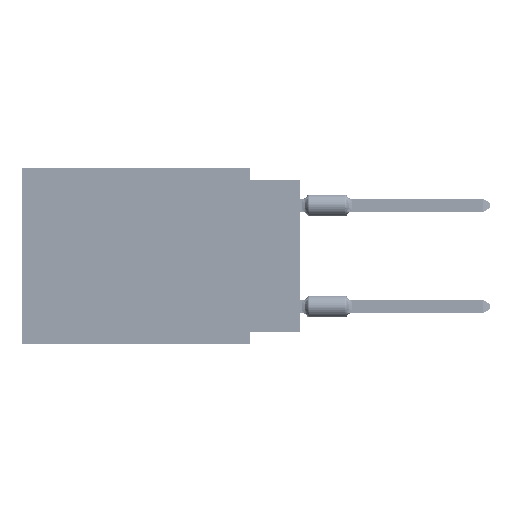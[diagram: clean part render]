
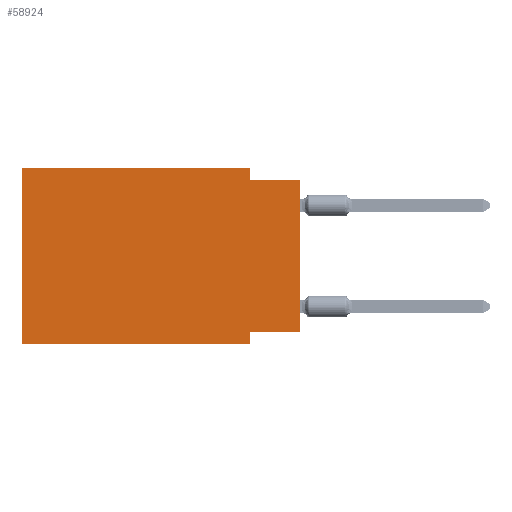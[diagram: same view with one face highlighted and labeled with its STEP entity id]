
A CAD part, left-side view. The second image highlights one B-rep face of the part: STEP entity #58924.
In plain terms, the highlighted planar face has unit normal (-1, 0, 0).
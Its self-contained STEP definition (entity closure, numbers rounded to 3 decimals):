
#3512 = LINE ( 'NONE', #9222, #46817 ) ;
#5720 = EDGE_CURVE ( 'NONE', #57578, #35784, #3512, .T. ) ;
#6951 = CARTESIAN_POINT ( 'NONE',  ( 0., 2.54, -8.255 ) ) ;
#9222 = CARTESIAN_POINT ( 'NONE',  ( 0., 2.54, -8.89 ) ) ;
#10628 = EDGE_LOOP ( 'NONE', ( #24085, #33129, #15882, #14444, #11402, #36207, #34136, #55691 ) ) ;
#11306 = VECTOR ( 'NONE', #19328, 1000. ) ;
#11402 = ORIENTED_EDGE ( 'NONE', *, *, #54731, .F. ) ;
#11644 = VERTEX_POINT ( 'NONE', #34146 ) ;
#11761 = CARTESIAN_POINT ( 'NONE',  ( 0., 13.97, -8.89 ) ) ;
#13430 = VERTEX_POINT ( 'NONE', #50425 ) ;
#13504 = DIRECTION ( 'NONE',  ( 0., -1., 0. ) ) ;
#13558 = VERTEX_POINT ( 'NONE', #47542 ) ;
#14444 = ORIENTED_EDGE ( 'NONE', *, *, #21468, .F. ) ;
#15882 = ORIENTED_EDGE ( 'NONE', *, *, #30518, .F. ) ;
#16103 = EDGE_CURVE ( 'NONE', #55023, #57578, #61866, .T. ) ;
#17272 = CARTESIAN_POINT ( 'NONE',  ( 0., 0., 0. ) ) ;
#17658 = DIRECTION ( 'NONE',  ( 0., -1., 0. ) ) ;
#19060 = EDGE_CURVE ( 'NONE', #11644, #13558, #30659, .T. ) ;
#19328 = DIRECTION ( 'NONE',  ( 0., 1., 0. ) ) ;
#19878 = VECTOR ( 'NONE', #59218, 1000. ) ;
#21468 = EDGE_CURVE ( 'NONE', #13430, #26968, #24415, .T. ) ;
#22025 = LINE ( 'NONE', #64933, #19878 ) ;
#23384 = PLANE ( 'NONE',  #51029 ) ;
#24085 = ORIENTED_EDGE ( 'NONE', *, *, #39243, .T. ) ;
#24415 = LINE ( 'NONE', #46201, #49723 ) ;
#25304 = DIRECTION ( 'NONE',  ( 0., 0., -1. ) ) ;
#26968 = VERTEX_POINT ( 'NONE', #33192 ) ;
#29818 = CARTESIAN_POINT ( 'NONE',  ( 0., 13.97, 0. ) ) ;
#30518 = EDGE_CURVE ( 'NONE', #26968, #11644, #49354, .T. ) ;
#30549 = CARTESIAN_POINT ( 'NONE',  ( 0., 0., -8.255 ) ) ;
#30659 = LINE ( 'NONE', #63192, #38471 ) ;
#33129 = ORIENTED_EDGE ( 'NONE', *, *, #19060, .F. ) ;
#33192 = CARTESIAN_POINT ( 'NONE',  ( 0., 2.54, 0. ) ) ;
#33758 = CARTESIAN_POINT ( 'NONE',  ( 0., 13.97, -8.89 ) ) ;
#34136 = ORIENTED_EDGE ( 'NONE', *, *, #5720, .F. ) ;
#34146 = CARTESIAN_POINT ( 'NONE',  ( 0., 2.54, -0.635 ) ) ;
#35784 = VERTEX_POINT ( 'NONE', #56295 ) ;
#36207 = ORIENTED_EDGE ( 'NONE', *, *, #49438, .T. ) ;
#38471 = VECTOR ( 'NONE', #13504, 1000. ) ;
#38616 = CARTESIAN_POINT ( 'NONE',  ( 0., 2.54, 0. ) ) ;
#39243 = EDGE_CURVE ( 'NONE', #55023, #13558, #44766, .T. ) ;
#42981 = VECTOR ( 'NONE', #17658, 1000. ) ;
#44766 = LINE ( 'NONE', #17272, #67908 ) ;
#45175 = DIRECTION ( 'NONE',  ( 1., 0., 0. ) ) ;
#46201 = CARTESIAN_POINT ( 'NONE',  ( 0., 13.97, 0. ) ) ;
#46817 = VECTOR ( 'NONE', #25304, 1000. ) ;
#47542 = CARTESIAN_POINT ( 'NONE',  ( 0., 0., -0.635 ) ) ;
#49354 = LINE ( 'NONE', #38616, #61385 ) ;
#49438 = EDGE_CURVE ( 'NONE', #62455, #35784, #65937, .T. ) ;
#49723 = VECTOR ( 'NONE', #68030, 1000. ) ;
#50425 = CARTESIAN_POINT ( 'NONE',  ( 0., 13.97, 0. ) ) ;
#51029 = AXIS2_PLACEMENT_3D ( 'NONE', #29818, #45175, #51270 ) ;
#51270 = DIRECTION ( 'NONE',  ( 0., 0., -1. ) ) ;
#54731 = EDGE_CURVE ( 'NONE', #62455, #13430, #22025, .T. ) ;
#55023 = VERTEX_POINT ( 'NONE', #30549 ) ;
#55691 = ORIENTED_EDGE ( 'NONE', *, *, #16103, .F. ) ;
#56295 = CARTESIAN_POINT ( 'NONE',  ( 0., 2.54, -8.89 ) ) ;
#57346 = FACE_OUTER_BOUND ( 'NONE', #10628, .T. ) ;
#57578 = VERTEX_POINT ( 'NONE', #6951 ) ;
#58924 = ADVANCED_FACE ( 'NONE', ( #57346 ), #23384, .F. ) ;
#59218 = DIRECTION ( 'NONE',  ( 0., 0., 1. ) ) ;
#60879 = DIRECTION ( 'NONE',  ( 0., 0., 1. ) ) ;
#61385 = VECTOR ( 'NONE', #65111, 1000. ) ;
#61866 = LINE ( 'NONE', #62572, #11306 ) ;
#62455 = VERTEX_POINT ( 'NONE', #11761 ) ;
#62572 = CARTESIAN_POINT ( 'NONE',  ( 0., 0., -8.255 ) ) ;
#63192 = CARTESIAN_POINT ( 'NONE',  ( 0., 0., -0.635 ) ) ;
#64933 = CARTESIAN_POINT ( 'NONE',  ( 0., 13.97, 0. ) ) ;
#65111 = DIRECTION ( 'NONE',  ( 0., 0., -1. ) ) ;
#65937 = LINE ( 'NONE', #33758, #42981 ) ;
#67908 = VECTOR ( 'NONE', #60879, 1000. ) ;
#68030 = DIRECTION ( 'NONE',  ( 0., -1., 0. ) ) ;
